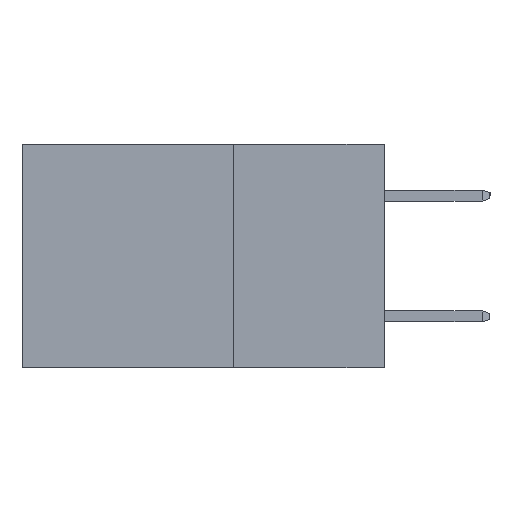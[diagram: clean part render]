
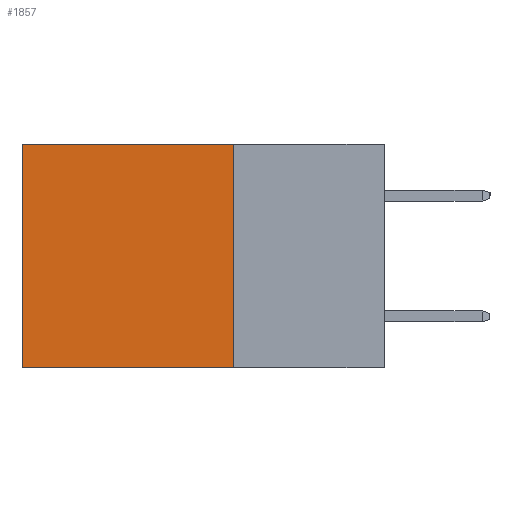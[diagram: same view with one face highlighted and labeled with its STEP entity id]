
A CAD part, left-side view. The second image highlights one B-rep face of the part: STEP entity #1857.
In plain terms, the highlighted planar face has unit normal (-1, 0, 0).
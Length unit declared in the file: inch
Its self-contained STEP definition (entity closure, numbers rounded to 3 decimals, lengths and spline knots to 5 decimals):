
#45 = EDGE_CURVE ( 'NONE', #14786, #14867, #14808, .T. ) ;
#1683 = ORIENTED_EDGE ( 'NONE', *, *, #12733, .F. ) ;
#1857 = ADVANCED_FACE ( 'NONE', ( #4487 ), #11614, .F. ) ;
#1936 = CARTESIAN_POINT ( 'NONE',  ( 0.2615, 0.25, -0.37 ) ) ;
#2120 = VECTOR ( 'NONE', #9759, 39.37008 ) ;
#3340 = CARTESIAN_POINT ( 'NONE',  ( 0.2615, 0.25, -0.37 ) ) ;
#3406 = DIRECTION ( 'NONE',  ( 0., 0., -1. ) ) ;
#3435 = CARTESIAN_POINT ( 'NONE',  ( 0.2615, 0.25, -0.37 ) ) ;
#3963 = CARTESIAN_POINT ( 'NONE',  ( 0.2615, 0.6, -0.37 ) ) ;
#4371 = ORIENTED_EDGE ( 'NONE', *, *, #4616, .F. ) ;
#4417 = LINE ( 'NONE', #7904, #10557 ) ;
#4487 = FACE_OUTER_BOUND ( 'NONE', #7322, .T. ) ;
#4616 = EDGE_CURVE ( 'NONE', #11910, #8509, #4417, .T. ) ;
#5537 = VECTOR ( 'NONE', #7527, 39.37008 ) ;
#5950 = CARTESIAN_POINT ( 'NONE',  ( 0.2615, 0.6, -0.37 ) ) ;
#6054 = AXIS2_PLACEMENT_3D ( 'NONE', #1936, #9223, #3406 ) ;
#6834 = LINE ( 'NONE', #3340, #14190 ) ;
#6884 = CARTESIAN_POINT ( 'NONE',  ( 0.2615, 0.6, 0. ) ) ;
#7135 = LINE ( 'NONE', #13010, #2120 ) ;
#7322 = EDGE_LOOP ( 'NONE', ( #11047, #1683, #4371, #9627 ) ) ;
#7527 = DIRECTION ( 'NONE',  ( 0., 0., -1. ) ) ;
#7904 = CARTESIAN_POINT ( 'NONE',  ( 0.2615, 0.25, -0.37 ) ) ;
#8509 = VERTEX_POINT ( 'NONE', #3435 ) ;
#9223 = DIRECTION ( 'NONE',  ( 1., 0., 0. ) ) ;
#9627 = ORIENTED_EDGE ( 'NONE', *, *, #11595, .T. ) ;
#9759 = DIRECTION ( 'NONE',  ( 0., 1., 0. ) ) ;
#10557 = VECTOR ( 'NONE', #14868, 39.37008 ) ;
#11047 = ORIENTED_EDGE ( 'NONE', *, *, #45, .T. ) ;
#11595 = EDGE_CURVE ( 'NONE', #11910, #14786, #7135, .T. ) ;
#11614 = PLANE ( 'NONE',  #6054 ) ;
#11910 = VERTEX_POINT ( 'NONE', #13362 ) ;
#12733 = EDGE_CURVE ( 'NONE', #8509, #14867, #6834, .T. ) ;
#13010 = CARTESIAN_POINT ( 'NONE',  ( 0.2615, 0.25, 0. ) ) ;
#13362 = CARTESIAN_POINT ( 'NONE',  ( 0.2615, 0.25, 0. ) ) ;
#14190 = VECTOR ( 'NONE', #15117, 39.37008 ) ;
#14786 = VERTEX_POINT ( 'NONE', #6884 ) ;
#14808 = LINE ( 'NONE', #3963, #5537 ) ;
#14867 = VERTEX_POINT ( 'NONE', #5950 ) ;
#14868 = DIRECTION ( 'NONE',  ( 0., 0., -1. ) ) ;
#15117 = DIRECTION ( 'NONE',  ( 0., 1., 0. ) ) ;
